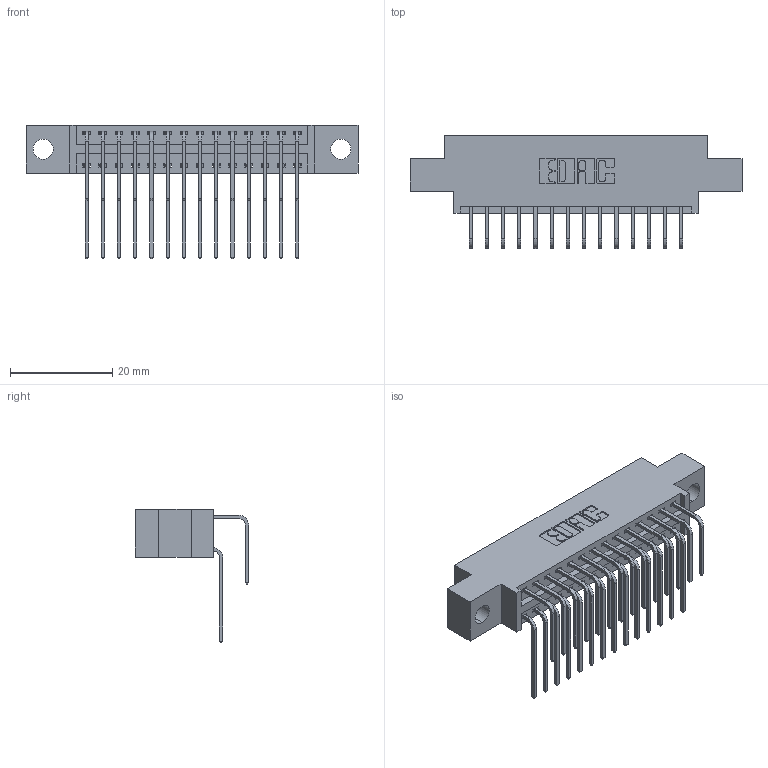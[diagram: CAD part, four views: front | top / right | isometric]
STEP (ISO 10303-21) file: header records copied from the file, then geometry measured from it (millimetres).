
FILE_DESCRIPTION (( 'STEP AP203' ), '1' );
FILE_NAME ('346-028-558-804.STEP', '2022-05-19T15:34:58', ( '' ), ( '' ), 'SwSTEP 2.0', 'SolidWorks 2020', '' );
FILE_SCHEMA (( 'CONFIG_CONTROL_DESIGN' ));
Length unit declared in the file: inch
Products named in the file (4): 345-292-001_558 559 Tail - 1; 345-292-001_558 Tail - 2; 346 Part_0.170 Offset - 0.156 Dia-TH; 346-028-558-804
Assembly tree (29 placements, depth 2):
  346-028-558-804
    346 Part_0.170 Offset - 0.156 Dia-TH
    345-292-001_558 559 Tail - 1  x14
    345-292-001_558 Tail - 2  x14
Bounding box: 65.02 x 22.16 x 26.16 mm (x, y, z)
Volume: 6024.1 mm3; surface area: 8642.9 mm2
Topology: 29 solids, 29 shells, 1652 faces, 4885 edges, 3218 vertices
Faces by surface type: plane 1130, cylinder 522
Entity records: 15241 total; most frequent: CARTESIAN_POINT 2609, ORIENTED_EDGE 2490, DIRECTION 2321, EDGE_CURVE 1245, LINE 1017, VECTOR 1017, VERTEX_POINT 826, AXIS2_PLACEMENT_3D 652
